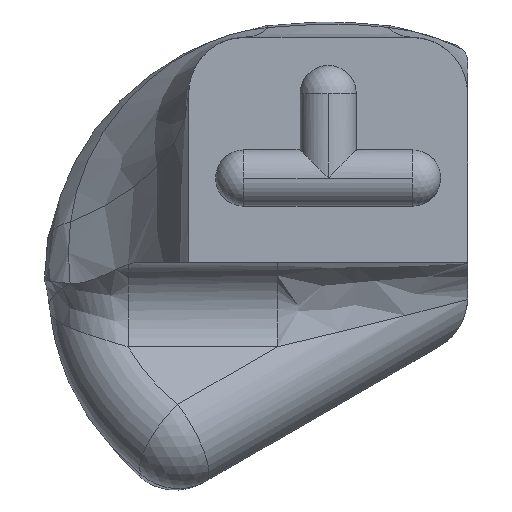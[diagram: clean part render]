
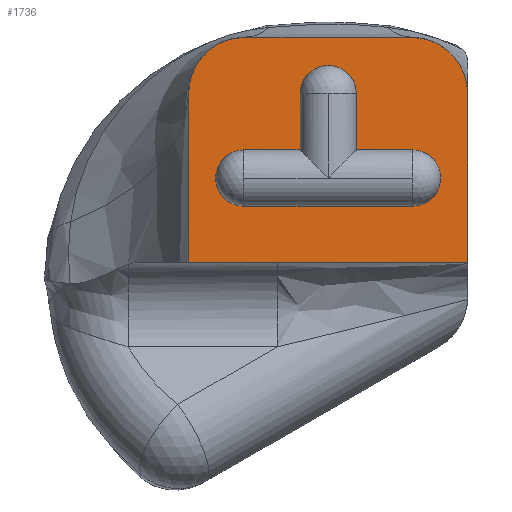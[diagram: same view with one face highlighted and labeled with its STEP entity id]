
A CAD part, left-side view. The second image highlights one B-rep face of the part: STEP entity #1736.
In plain terms, the highlighted planar face has unit normal (-1, 0, 0).
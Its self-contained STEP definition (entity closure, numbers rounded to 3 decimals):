
#27 = FACE_BOUND ( 'NONE', #1790, .T. ) ;
#29 = EDGE_CURVE ( 'NONE', #1133, #1710, #1201, .T. ) ;
#56 = DIRECTION ( 'NONE',  ( 0., -0.5, -0.866 ) ) ;
#62 = DIRECTION ( 'NONE',  ( -1., 0., 0. ) ) ;
#78 = CARTESIAN_POINT ( 'NONE',  ( 10.292, 14.9, -10. ) ) ;
#81 = CARTESIAN_POINT ( 'NONE',  ( 10.292, 0., -20. ) ) ;
#111 = EDGE_LOOP ( 'NONE', ( #1182, #1242, #465, #1440, #832, #512 ) ) ;
#114 = VERTEX_POINT ( 'NONE', #1095 ) ;
#133 = EDGE_CURVE ( 'NONE', #600, #647, #1146, .T. ) ;
#172 = LINE ( 'NONE', #1059, #1731 ) ;
#173 = LINE ( 'NONE', #1163, #326 ) ;
#187 = CARTESIAN_POINT ( 'NONE',  ( 10.292, 9.9, -48.117 ) ) ;
#230 = VECTOR ( 'NONE', #1203, 1000. ) ;
#255 = CARTESIAN_POINT ( 'NONE',  ( 10.292, 19.9, -12.5 ) ) ;
#268 = CARTESIAN_POINT ( 'NONE',  ( 10.292, 9.9, -10. ) ) ;
#289 = VECTOR ( 'NONE', #1679, 1000. ) ;
#310 = DIRECTION ( 'NONE',  ( 0., 0., 1. ) ) ;
#314 = CARTESIAN_POINT ( 'NONE',  ( 10.292, 4.9, -10. ) ) ;
#326 = VECTOR ( 'NONE', #1316, 1000. ) ;
#378 = CARTESIAN_POINT ( 'NONE',  ( 10.292, 24.8, -20. ) ) ;
#397 = LINE ( 'NONE', #1549, #289 ) ;
#404 = DIRECTION ( 'NONE',  ( 0., -0.5, -0.866 ) ) ;
#405 = CARTESIAN_POINT ( 'NONE',  ( 10.292, 12.4, -20. ) ) ;
#409 = DIRECTION ( 'NONE',  ( 1., 0., 0. ) ) ;
#415 = LINE ( 'NONE', #187, #1560 ) ;
#419 = CARTESIAN_POINT ( 'NONE',  ( 10.292, 19.9, -10. ) ) ;
#444 = DIRECTION ( 'NONE',  ( -1., 0., 0. ) ) ;
#447 = CIRCLE ( 'NONE', #483, 5. ) ;
#458 = CARTESIAN_POINT ( 'NONE',  ( 10.292, 24.8, -5. ) ) ;
#465 = ORIENTED_EDGE ( 'NONE', *, *, #1758, .T. ) ;
#476 = AXIS2_PLACEMENT_3D ( 'NONE', #255, #1300, #404 ) ;
#478 = VERTEX_POINT ( 'NONE', #419 ) ;
#483 = AXIS2_PLACEMENT_3D ( 'NONE', #542, #1597, #691 ) ;
#495 = CIRCLE ( 'NONE', #476, 2.5 ) ;
#508 = CARTESIAN_POINT ( 'NONE',  ( 10.292, 14.9, -48.117 ) ) ;
#512 = ORIENTED_EDGE ( 'NONE', *, *, #1400, .T. ) ;
#531 = CARTESIAN_POINT ( 'NONE',  ( 10.292, 9.9, -5. ) ) ;
#542 = CARTESIAN_POINT ( 'NONE',  ( 10.292, 19.8, -5. ) ) ;
#584 = VERTEX_POINT ( 'NONE', #268 ) ;
#600 = VERTEX_POINT ( 'NONE', #892 ) ;
#647 = VERTEX_POINT ( 'NONE', #314 ) ;
#663 = CIRCLE ( 'NONE', #978, 2.5 ) ;
#675 = AXIS2_PLACEMENT_3D ( 'NONE', #1344, #444, #1503 ) ;
#691 = DIRECTION ( 'NONE',  ( 0., 0.5, 0.866 ) ) ;
#699 = FACE_OUTER_BOUND ( 'NONE', #111, .T. ) ;
#732 = VERTEX_POINT ( 'NONE', #1024 ) ;
#747 = CARTESIAN_POINT ( 'NONE',  ( 10.292, 12.4, -5. ) ) ;
#748 = EDGE_CURVE ( 'NONE', #754, #600, #1148, .T. ) ;
#754 = VERTEX_POINT ( 'NONE', #898 ) ;
#781 = AXIS2_PLACEMENT_3D ( 'NONE', #1439, #409, #1470 ) ;
#807 = CARTESIAN_POINT ( 'NONE',  ( 10.292, 32.021, -10. ) ) ;
#832 = ORIENTED_EDGE ( 'NONE', *, *, #1721, .T. ) ;
#853 = CARTESIAN_POINT ( 'NONE',  ( 10.292, 19.8, 0. ) ) ;
#892 = CARTESIAN_POINT ( 'NONE',  ( 10.292, 4.9, -15. ) ) ;
#894 = DIRECTION ( 'NONE',  ( 0., -0.5, -0.866 ) ) ;
#898 = CARTESIAN_POINT ( 'NONE',  ( 10.292, 19.9, -15. ) ) ;
#951 = ORIENTED_EDGE ( 'NONE', *, *, #1471, .T. ) ;
#960 = DIRECTION ( 'NONE',  ( 0., -1., 0. ) ) ;
#978 = AXIS2_PLACEMENT_3D ( 'NONE', #747, #1764, #894 ) ;
#1022 = VERTEX_POINT ( 'NONE', #78 ) ;
#1024 = CARTESIAN_POINT ( 'NONE',  ( 10.292, 5., 0. ) ) ;
#1059 = CARTESIAN_POINT ( 'NONE',  ( 10.292, 0., -214.388 ) ) ;
#1071 = ORIENTED_EDGE ( 'NONE', *, *, #1217, .F. ) ;
#1091 = LINE ( 'NONE', #1194, #230 ) ;
#1095 = CARTESIAN_POINT ( 'NONE',  ( 10.292, 14.9, -5. ) ) ;
#1113 = ORIENTED_EDGE ( 'NONE', *, *, #1450, .F. ) ;
#1130 = ORIENTED_EDGE ( 'NONE', *, *, #133, .F. ) ;
#1133 = VERTEX_POINT ( 'NONE', #81 ) ;
#1146 = CIRCLE ( 'NONE', #1235, 2.5 ) ;
#1148 = LINE ( 'NONE', #1526, #1392 ) ;
#1156 = PLANE ( 'NONE',  #781 ) ;
#1163 = CARTESIAN_POINT ( 'NONE',  ( 10.292, 32.021, -10. ) ) ;
#1182 = ORIENTED_EDGE ( 'NONE', *, *, #29, .F. ) ;
#1194 = CARTESIAN_POINT ( 'NONE',  ( 10.292, 24.8, -214.388 ) ) ;
#1201 = LINE ( 'NONE', #405, #1543 ) ;
#1203 = DIRECTION ( 'NONE',  ( 0., 0., -1. ) ) ;
#1214 = DIRECTION ( 'NONE',  ( 0., 1., 0. ) ) ;
#1217 = EDGE_CURVE ( 'NONE', #478, #754, #495, .T. ) ;
#1235 = AXIS2_PLACEMENT_3D ( 'NONE', #1557, #62, #56 ) ;
#1242 = ORIENTED_EDGE ( 'NONE', *, *, #1781, .T. ) ;
#1250 = VERTEX_POINT ( 'NONE', #853 ) ;
#1283 = LINE ( 'NONE', #807, #1301 ) ;
#1300 = DIRECTION ( 'NONE',  ( -1., 0., 0. ) ) ;
#1301 = VECTOR ( 'NONE', #960, 1000. ) ;
#1316 = DIRECTION ( 'NONE',  ( 0., -1., 0. ) ) ;
#1344 = CARTESIAN_POINT ( 'NONE',  ( 10.292, 5., -5. ) ) ;
#1371 = CARTESIAN_POINT ( 'NONE',  ( 10.292, 0., -5. ) ) ;
#1377 = ORIENTED_EDGE ( 'NONE', *, *, #1760, .F. ) ;
#1385 = ORIENTED_EDGE ( 'NONE', *, *, #1490, .T. ) ;
#1392 = VECTOR ( 'NONE', #1645, 1000. ) ;
#1400 = EDGE_CURVE ( 'NONE', #1406, #1710, #1091, .T. ) ;
#1406 = VERTEX_POINT ( 'NONE', #458 ) ;
#1412 = VECTOR ( 'NONE', #1564, 1000. ) ;
#1415 = CIRCLE ( 'NONE', #675, 5. ) ;
#1439 = CARTESIAN_POINT ( 'NONE',  ( 10.292, -48.551, -288.347 ) ) ;
#1440 = ORIENTED_EDGE ( 'NONE', *, *, #1869, .T. ) ;
#1450 = EDGE_CURVE ( 'NONE', #584, #1734, #415, .T. ) ;
#1470 = DIRECTION ( 'NONE',  ( 0., 0.5, 0.866 ) ) ;
#1471 = EDGE_CURVE ( 'NONE', #1022, #114, #1831, .T. ) ;
#1490 = EDGE_CURVE ( 'NONE', #478, #1022, #1283, .T. ) ;
#1503 = DIRECTION ( 'NONE',  ( 0., 0.5, 0.866 ) ) ;
#1522 = DIRECTION ( 'NONE',  ( 0., 0., 1. ) ) ;
#1526 = CARTESIAN_POINT ( 'NONE',  ( 10.292, 32.021, -15. ) ) ;
#1543 = VECTOR ( 'NONE', #1214, 1000. ) ;
#1549 = CARTESIAN_POINT ( 'NONE',  ( 10.292, 12.4, 0. ) ) ;
#1557 = CARTESIAN_POINT ( 'NONE',  ( 10.292, 4.9, -12.5 ) ) ;
#1560 = VECTOR ( 'NONE', #1522, 1000. ) ;
#1564 = DIRECTION ( 'NONE',  ( 0., 0., 1. ) ) ;
#1597 = DIRECTION ( 'NONE',  ( -1., 0., 0. ) ) ;
#1645 = DIRECTION ( 'NONE',  ( 0., -1., 0. ) ) ;
#1679 = DIRECTION ( 'NONE',  ( 0., 1., 0. ) ) ;
#1710 = VERTEX_POINT ( 'NONE', #378 ) ;
#1721 = EDGE_CURVE ( 'NONE', #1250, #1406, #447, .T. ) ;
#1731 = VECTOR ( 'NONE', #310, 1000. ) ;
#1734 = VERTEX_POINT ( 'NONE', #531 ) ;
#1736 = ADVANCED_FACE ( 'NONE', ( #27, #699 ), #1156, .F. ) ;
#1751 = EDGE_CURVE ( 'NONE', #584, #647, #173, .T. ) ;
#1758 = EDGE_CURVE ( 'NONE', #1825, #732, #1415, .T. ) ;
#1760 = EDGE_CURVE ( 'NONE', #1734, #114, #663, .T. ) ;
#1764 = DIRECTION ( 'NONE',  ( -1., 0., 0. ) ) ;
#1781 = EDGE_CURVE ( 'NONE', #1133, #1825, #172, .T. ) ;
#1790 = EDGE_LOOP ( 'NONE', ( #1385, #951, #1377, #1113, #1850, #1130, #1817, #1071 ) ) ;
#1817 = ORIENTED_EDGE ( 'NONE', *, *, #748, .F. ) ;
#1825 = VERTEX_POINT ( 'NONE', #1371 ) ;
#1831 = LINE ( 'NONE', #508, #1412 ) ;
#1850 = ORIENTED_EDGE ( 'NONE', *, *, #1751, .T. ) ;
#1869 = EDGE_CURVE ( 'NONE', #732, #1250, #397, .T. ) ;
